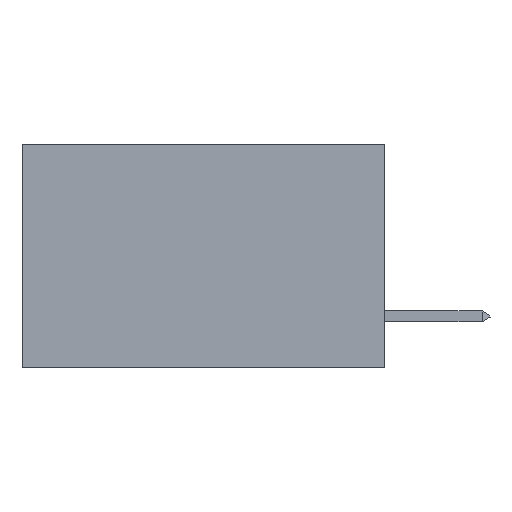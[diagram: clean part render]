
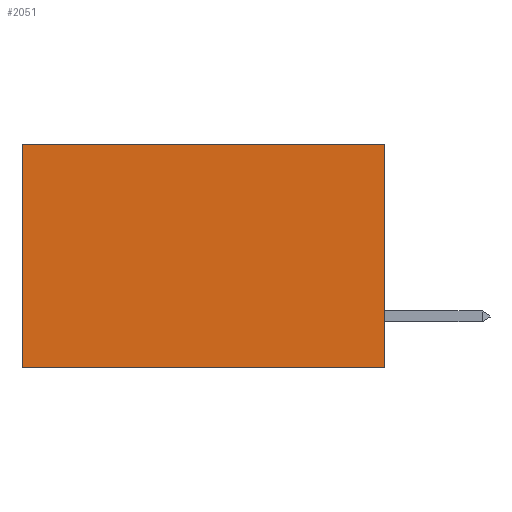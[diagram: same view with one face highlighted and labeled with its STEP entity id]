
A CAD part, left-side view. The second image highlights one B-rep face of the part: STEP entity #2051.
In plain terms, the highlighted planar face has unit normal (-1, 0, 0).
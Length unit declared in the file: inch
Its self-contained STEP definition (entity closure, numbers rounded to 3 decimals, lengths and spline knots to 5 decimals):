
#206 = DIRECTION ( 'NONE',  ( 0., 0., -1. ) ) ;
#265 = EDGE_CURVE ( 'NONE', #8262, #12027, #727, .T. ) ;
#425 = AXIS2_PLACEMENT_3D ( 'NONE', #2783, #7592, #13421 ) ;
#547 = LINE ( 'NONE', #8865, #5505 ) ;
#727 = LINE ( 'NONE', #12558, #12188 ) ;
#1423 = CARTESIAN_POINT ( 'NONE',  ( 0.2875, 0.6, 0. ) ) ;
#2001 = ORIENTED_EDGE ( 'NONE', *, *, #265, .F. ) ;
#2051 = ADVANCED_FACE ( 'NONE', ( #12136 ), #14832, .F. ) ;
#2547 = VERTEX_POINT ( 'NONE', #1423 ) ;
#2708 = CARTESIAN_POINT ( 'NONE',  ( 0.2875, 0., -0.37 ) ) ;
#2783 = CARTESIAN_POINT ( 'NONE',  ( 0.2875, 0., 0. ) ) ;
#3543 = CARTESIAN_POINT ( 'NONE',  ( 0.2875, 0., 0. ) ) ;
#3639 = LINE ( 'NONE', #9143, #11471 ) ;
#3700 = ORIENTED_EDGE ( 'NONE', *, *, #9987, .F. ) ;
#4238 = EDGE_CURVE ( 'NONE', #2547, #8533, #10773, .T. ) ;
#4666 = ORIENTED_EDGE ( 'NONE', *, *, #4238, .T. ) ;
#5350 = ORIENTED_EDGE ( 'NONE', *, *, #9866, .T. ) ;
#5467 = DIRECTION ( 'NONE',  ( 0., 0., -1. ) ) ;
#5505 = VECTOR ( 'NONE', #11262, 39.37008 ) ;
#5684 = CARTESIAN_POINT ( 'NONE',  ( 0.2875, 0.6, 0. ) ) ;
#7592 = DIRECTION ( 'NONE',  ( 1., 0., 0. ) ) ;
#7601 = VECTOR ( 'NONE', #206, 39.37008 ) ;
#7780 = CARTESIAN_POINT ( 'NONE',  ( 0.2875, 0.6, -0.37 ) ) ;
#7949 = EDGE_LOOP ( 'NONE', ( #4666, #3700, #2001, #5350 ) ) ;
#8262 = VERTEX_POINT ( 'NONE', #3543 ) ;
#8533 = VERTEX_POINT ( 'NONE', #7780 ) ;
#8865 = CARTESIAN_POINT ( 'NONE',  ( 0.2875, 0., 0. ) ) ;
#9143 = CARTESIAN_POINT ( 'NONE',  ( 0.2875, 0., -0.37 ) ) ;
#9866 = EDGE_CURVE ( 'NONE', #8262, #2547, #547, .T. ) ;
#9987 = EDGE_CURVE ( 'NONE', #12027, #8533, #3639, .T. ) ;
#10773 = LINE ( 'NONE', #5684, #7601 ) ;
#11262 = DIRECTION ( 'NONE',  ( 0., 1., 0. ) ) ;
#11471 = VECTOR ( 'NONE', #13773, 39.37008 ) ;
#12027 = VERTEX_POINT ( 'NONE', #2708 ) ;
#12136 = FACE_OUTER_BOUND ( 'NONE', #7949, .T. ) ;
#12188 = VECTOR ( 'NONE', #5467, 39.37008 ) ;
#12558 = CARTESIAN_POINT ( 'NONE',  ( 0.2875, 0., 0. ) ) ;
#13421 = DIRECTION ( 'NONE',  ( 0., 0., -1. ) ) ;
#13773 = DIRECTION ( 'NONE',  ( 0., 1., 0. ) ) ;
#14832 = PLANE ( 'NONE',  #425 ) ;
